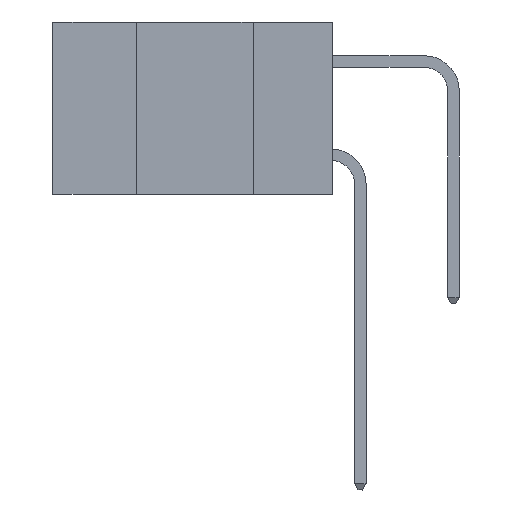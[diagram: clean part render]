
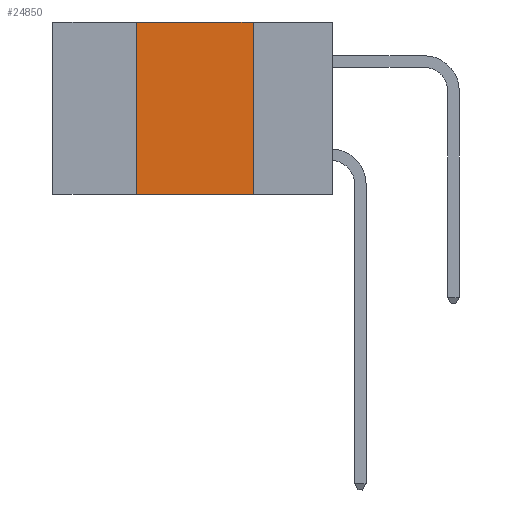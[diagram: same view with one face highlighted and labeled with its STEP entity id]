
A CAD part, left-side view. The second image highlights one B-rep face of the part: STEP entity #24850.
In plain terms, the highlighted planar face has unit normal (-1, 0, 0).
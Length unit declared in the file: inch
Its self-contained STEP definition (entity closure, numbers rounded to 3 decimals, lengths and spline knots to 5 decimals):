
#2580 = CARTESIAN_POINT ( 'NONE',  ( 0., 0.17, -0.37 ) ) ;
#3034 = DIRECTION ( 'NONE',  ( 0., 0., 1. ) ) ;
#4318 = VECTOR ( 'NONE', #5539, 39.37008 ) ;
#4659 = ORIENTED_EDGE ( 'NONE', *, *, #7878, .F. ) ;
#4998 = DIRECTION ( 'NONE',  ( 0., -1., 0. ) ) ;
#5539 = DIRECTION ( 'NONE',  ( 0., 0., -1. ) ) ;
#7107 = VERTEX_POINT ( 'NONE', #24673 ) ;
#7136 = PLANE ( 'NONE',  #10671 ) ;
#7878 = EDGE_CURVE ( 'NONE', #20346, #7107, #30898, .T. ) ;
#7946 = CARTESIAN_POINT ( 'NONE',  ( 0., 0.17, 0. ) ) ;
#8212 = EDGE_CURVE ( 'NONE', #7107, #25013, #30455, .T. ) ;
#9895 = DIRECTION ( 'NONE',  ( 0., -1., 0. ) ) ;
#9981 = CARTESIAN_POINT ( 'NONE',  ( 0., 0.6, 0. ) ) ;
#10013 = CARTESIAN_POINT ( 'NONE',  ( 0., 0.6, -0.37 ) ) ;
#10671 = AXIS2_PLACEMENT_3D ( 'NONE', #9981, #17643, #27786 ) ;
#12062 = CARTESIAN_POINT ( 'NONE',  ( 0., 0.42, -0.37 ) ) ;
#12128 = LINE ( 'NONE', #10013, #18676 ) ;
#12692 = VERTEX_POINT ( 'NONE', #12062 ) ;
#12762 = EDGE_CURVE ( 'NONE', #12692, #25013, #12128, .T. ) ;
#12958 = VECTOR ( 'NONE', #3034, 39.37008 ) ;
#14683 = CARTESIAN_POINT ( 'NONE',  ( 0., 0.6, 0. ) ) ;
#14698 = EDGE_LOOP ( 'NONE', ( #31198, #4659, #22323, #26746 ) ) ;
#17527 = FACE_OUTER_BOUND ( 'NONE', #14698, .T. ) ;
#17643 = DIRECTION ( 'NONE',  ( 1., 0., 0. ) ) ;
#18676 = VECTOR ( 'NONE', #4998, 39.37008 ) ;
#20346 = VERTEX_POINT ( 'NONE', #32170 ) ;
#22323 = ORIENTED_EDGE ( 'NONE', *, *, #33161, .F. ) ;
#24673 = CARTESIAN_POINT ( 'NONE',  ( 0., 0.17, 0. ) ) ;
#24850 = ADVANCED_FACE ( 'NONE', ( #17527 ), #7136, .F. ) ;
#25013 = VERTEX_POINT ( 'NONE', #2580 ) ;
#26725 = VECTOR ( 'NONE', #9895, 39.37008 ) ;
#26746 = ORIENTED_EDGE ( 'NONE', *, *, #12762, .T. ) ;
#27786 = DIRECTION ( 'NONE',  ( 0., 0., -1. ) ) ;
#28493 = LINE ( 'NONE', #28941, #12958 ) ;
#28941 = CARTESIAN_POINT ( 'NONE',  ( 0., 0.42, 0. ) ) ;
#30455 = LINE ( 'NONE', #7946, #4318 ) ;
#30898 = LINE ( 'NONE', #14683, #26725 ) ;
#31198 = ORIENTED_EDGE ( 'NONE', *, *, #8212, .F. ) ;
#32170 = CARTESIAN_POINT ( 'NONE',  ( 0., 0.42, 0. ) ) ;
#33161 = EDGE_CURVE ( 'NONE', #12692, #20346, #28493, .T. ) ;
